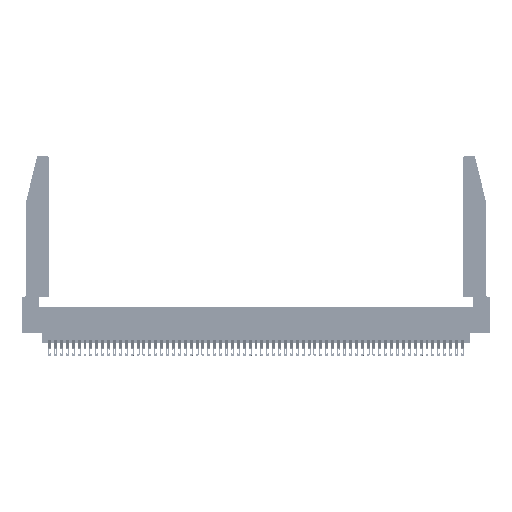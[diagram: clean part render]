
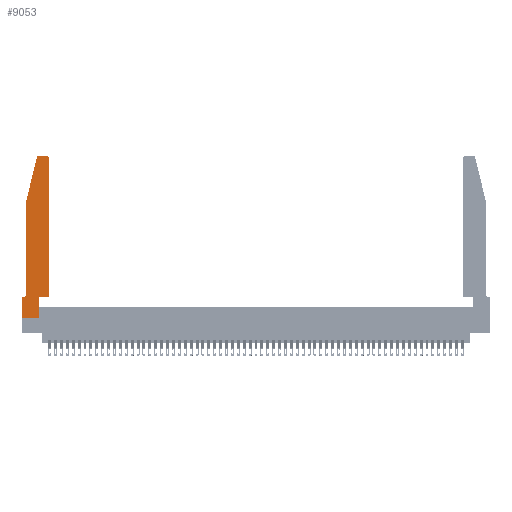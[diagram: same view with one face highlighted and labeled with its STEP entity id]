
A CAD part, top view. The second image highlights one B-rep face of the part: STEP entity #9053.
In plain terms, the highlighted planar face has unit normal (0, 0, 1).
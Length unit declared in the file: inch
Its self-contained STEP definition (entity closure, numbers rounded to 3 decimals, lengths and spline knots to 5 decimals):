
#227 = CIRCLE ( 'NONE', #50838, 0.03 ) ;
#1637 = CARTESIAN_POINT ( 'NONE',  ( 0.0755, 0.35, 0.37 ) ) ;
#2494 = EDGE_CURVE ( 'NONE', #30972, #35377, #52343, .T. ) ;
#2616 = EDGE_CURVE ( 'NONE', #43484, #34285, #48159, .T. ) ;
#2999 = EDGE_CURVE ( 'NONE', #24778, #52513, #41285, .T. ) ;
#3832 = DIRECTION ( 'NONE',  ( 0., 1., 0. ) ) ;
#4093 = DIRECTION ( 'NONE',  ( 1., 0., 0. ) ) ;
#4111 = DIRECTION ( 'NONE',  ( -0.239, -0.971, 0. ) ) ;
#4222 = CARTESIAN_POINT ( 'NONE',  ( 0.0055, 0.42, 0.37 ) ) ;
#4878 = DIRECTION ( 'NONE',  ( 1., 0., 0. ) ) ;
#5236 = ORIENTED_EDGE ( 'NONE', *, *, #52610, .T. ) ;
#5240 = LINE ( 'NONE', #53197, #49331 ) ;
#6211 = DIRECTION ( 'NONE',  ( 0., -1., 0. ) ) ;
#6215 = EDGE_CURVE ( 'NONE', #34285, #18100, #30609, .T. ) ;
#6320 = EDGE_CURVE ( 'NONE', #53258, #11306, #227, .T. ) ;
#6382 = DIRECTION ( 'NONE',  ( 1., 0., 0. ) ) ;
#6422 = ORIENTED_EDGE ( 'NONE', *, *, #6320, .T. ) ;
#6576 = DIRECTION ( 'NONE',  ( 1., 0., 0. ) ) ;
#7144 = CARTESIAN_POINT ( 'NONE',  ( 0., 0.35, 0.37 ) ) ;
#7225 = CARTESIAN_POINT ( 'NONE',  ( 0.2865, 0., 0.37 ) ) ;
#7745 = VECTOR ( 'NONE', #50536, 39.37008 ) ;
#8420 = CARTESIAN_POINT ( 'NONE',  ( 0.2865, 0.35, 0.37 ) ) ;
#8839 = DIRECTION ( 'NONE',  ( 0., 0., -1. ) ) ;
#9053 = ADVANCED_FACE ( 'NONE', ( #52259 ), #16007, .T. ) ;
#9126 = ORIENTED_EDGE ( 'NONE', *, *, #47591, .T. ) ;
#9799 = ORIENTED_EDGE ( 'NONE', *, *, #29580, .T. ) ;
#11306 = VERTEX_POINT ( 'NONE', #48215 ) ;
#11446 = AXIS2_PLACEMENT_3D ( 'NONE', #55050, #46413, #6382 ) ;
#11512 = DIRECTION ( 'NONE',  ( 1., 0., 0. ) ) ;
#13115 = DIRECTION ( 'NONE',  ( -1., 0., 0. ) ) ;
#13547 = DIRECTION ( 'NONE',  ( 0., 0., 1. ) ) ;
#14277 = DIRECTION ( 'NONE',  ( -1., 0., 0. ) ) ;
#14649 = CARTESIAN_POINT ( 'NONE',  ( 0.0055, 0.35, 0.37 ) ) ;
#16007 = PLANE ( 'NONE',  #11446 ) ;
#16690 = EDGE_CURVE ( 'NONE', #21060, #54662, #5240, .T. ) ;
#16935 = ORIENTED_EDGE ( 'NONE', *, *, #32872, .T. ) ;
#17052 = EDGE_LOOP ( 'NONE', ( #5236, #9799, #33327, #35823, #43811, #9126, #36715, #17130, #42229, #37848, #16935, #6422 ) ) ;
#17130 = ORIENTED_EDGE ( 'NONE', *, *, #6215, .T. ) ;
#18100 = VERTEX_POINT ( 'NONE', #7225 ) ;
#19811 = LINE ( 'NONE', #1637, #21204 ) ;
#20566 = CARTESIAN_POINT ( 'NONE',  ( 0.4505, 0.35, 0.37 ) ) ;
#21060 = VERTEX_POINT ( 'NONE', #27457 ) ;
#21204 = VECTOR ( 'NONE', #28437, 39.37008 ) ;
#23640 = EDGE_CURVE ( 'NONE', #54662, #30972, #53832, .T. ) ;
#24778 = VERTEX_POINT ( 'NONE', #8420 ) ;
#25039 = CIRCLE ( 'NONE', #54530, 0.03 ) ;
#26317 = VECTOR ( 'NONE', #6211, 39.37008 ) ;
#27457 = CARTESIAN_POINT ( 'NONE',  ( 0.25487, 2.72718, 0.37 ) ) ;
#27508 = VECTOR ( 'NONE', #35033, 39.37008 ) ;
#28437 = DIRECTION ( 'NONE',  ( -1., 0., 0. ) ) ;
#29580 = EDGE_CURVE ( 'NONE', #37886, #21060, #25039, .T. ) ;
#30260 = VECTOR ( 'NONE', #3832, 39.37008 ) ;
#30440 = CARTESIAN_POINT ( 'NONE',  ( 0., 0., 0.37 ) ) ;
#30609 = LINE ( 'NONE', #45119, #43009 ) ;
#30972 = VERTEX_POINT ( 'NONE', #32258 ) ;
#30993 = VECTOR ( 'NONE', #11512, 39.37008 ) ;
#31299 = VECTOR ( 'NONE', #14277, 39.37008 ) ;
#32258 = CARTESIAN_POINT ( 'NONE',  ( 0.0755, 0.42, 0.37 ) ) ;
#32872 = EDGE_CURVE ( 'NONE', #52513, #53258, #43992, .T. ) ;
#33327 = ORIENTED_EDGE ( 'NONE', *, *, #16690, .T. ) ;
#34285 = VERTEX_POINT ( 'NONE', #38743 ) ;
#35033 = DIRECTION ( 'NONE',  ( 0., -1., 0. ) ) ;
#35377 = VERTEX_POINT ( 'NONE', #14649 ) ;
#35823 = ORIENTED_EDGE ( 'NONE', *, *, #23640, .T. ) ;
#36122 = LINE ( 'NONE', #44886, #31299 ) ;
#36715 = ORIENTED_EDGE ( 'NONE', *, *, #2616, .T. ) ;
#37212 = CARTESIAN_POINT ( 'NONE',  ( 0.284, 2.75, 0.37 ) ) ;
#37377 = DIRECTION ( 'NONE',  ( 0., 0., 1. ) ) ;
#37848 = ORIENTED_EDGE ( 'NONE', *, *, #2999, .T. ) ;
#37886 = VERTEX_POINT ( 'NONE', #37212 ) ;
#38743 = CARTESIAN_POINT ( 'NONE',  ( 0., 0., 0.37 ) ) ;
#39871 = CARTESIAN_POINT ( 'NONE',  ( 0.4505, 0.35, 0.37 ) ) ;
#39902 = CARTESIAN_POINT ( 'NONE',  ( 0.284, 2.72, 0.37 ) ) ;
#41285 = LINE ( 'NONE', #20566, #30993 ) ;
#41444 = CARTESIAN_POINT ( 'NONE',  ( 0.2865, 0.35, 0.37 ) ) ;
#41798 = CARTESIAN_POINT ( 'NONE',  ( 0.0755, 2., 0.37 ) ) ;
#42229 = ORIENTED_EDGE ( 'NONE', *, *, #53693, .T. ) ;
#42763 = CARTESIAN_POINT ( 'NONE',  ( 0.4505, 2.72, 0.37 ) ) ;
#42975 = AXIS2_PLACEMENT_3D ( 'NONE', #4222, #8839, #13115 ) ;
#43009 = VECTOR ( 'NONE', #4878, 39.37008 ) ;
#43484 = VERTEX_POINT ( 'NONE', #7144 ) ;
#43811 = ORIENTED_EDGE ( 'NONE', *, *, #2494, .T. ) ;
#43992 = LINE ( 'NONE', #56755, #30260 ) ;
#44886 = CARTESIAN_POINT ( 'NONE',  ( 0.2605, 2.75, 0.37 ) ) ;
#45119 = CARTESIAN_POINT ( 'NONE',  ( 0., 0., 0.37 ) ) ;
#46413 = DIRECTION ( 'NONE',  ( 0., 0., 1. ) ) ;
#47591 = EDGE_CURVE ( 'NONE', #35377, #43484, #19811, .T. ) ;
#48159 = LINE ( 'NONE', #30440, #27508 ) ;
#48215 = CARTESIAN_POINT ( 'NONE',  ( 0.4205, 2.75, 0.37 ) ) ;
#48493 = CARTESIAN_POINT ( 'NONE',  ( 0.0755, 2., 0.37 ) ) ;
#49331 = VECTOR ( 'NONE', #4111, 39.37008 ) ;
#49803 = LINE ( 'NONE', #41444, #7745 ) ;
#50536 = DIRECTION ( 'NONE',  ( 0., 1., 0. ) ) ;
#50838 = AXIS2_PLACEMENT_3D ( 'NONE', #55242, #37377, #6576 ) ;
#52259 = FACE_OUTER_BOUND ( 'NONE', #17052, .T. ) ;
#52343 = CIRCLE ( 'NONE', #42975, 0.07 ) ;
#52513 = VERTEX_POINT ( 'NONE', #39871 ) ;
#52610 = EDGE_CURVE ( 'NONE', #11306, #37886, #36122, .T. ) ;
#53197 = CARTESIAN_POINT ( 'NONE',  ( 0.0755, 2., 0.37 ) ) ;
#53258 = VERTEX_POINT ( 'NONE', #42763 ) ;
#53693 = EDGE_CURVE ( 'NONE', #18100, #24778, #49803, .T. ) ;
#53832 = LINE ( 'NONE', #41798, #26317 ) ;
#54530 = AXIS2_PLACEMENT_3D ( 'NONE', #39902, #13547, #4093 ) ;
#54662 = VERTEX_POINT ( 'NONE', #48493 ) ;
#55050 = CARTESIAN_POINT ( 'NONE',  ( 0., 0.35, 0.37 ) ) ;
#55242 = CARTESIAN_POINT ( 'NONE',  ( 0.4205, 2.72, 0.37 ) ) ;
#56755 = CARTESIAN_POINT ( 'NONE',  ( 0.4505, 0.35, 0.37 ) ) ;
